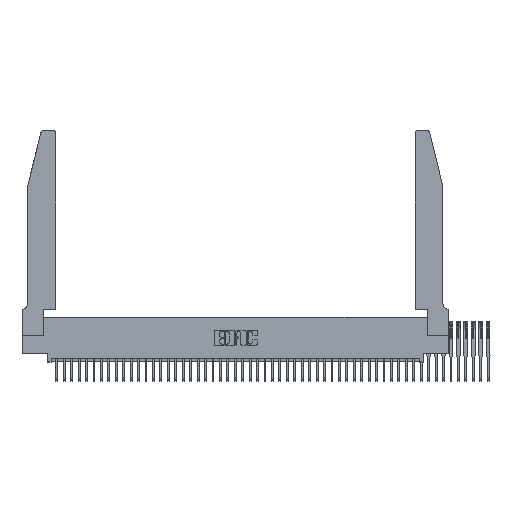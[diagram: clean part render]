
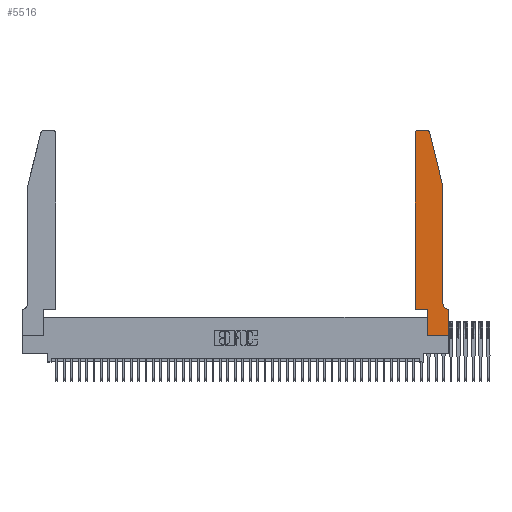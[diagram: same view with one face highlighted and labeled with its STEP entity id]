
A CAD part, top view. The second image highlights one B-rep face of the part: STEP entity #5516.
In plain terms, the highlighted face is planar.
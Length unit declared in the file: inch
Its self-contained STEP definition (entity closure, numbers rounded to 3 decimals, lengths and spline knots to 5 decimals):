
#220 = VERTEX_POINT ( 'NONE', #24858 ) ;
#544 = VERTEX_POINT ( 'NONE', #23576 ) ;
#2087 = EDGE_CURVE ( 'NONE', #5061, #9962, #10847, .T. ) ;
#2173 = DIRECTION ( 'NONE',  ( -1., 0., 0. ) ) ;
#2251 = CARTESIAN_POINT ( 'NONE',  ( 0.4505, 0.35, 0. ) ) ;
#2755 = VECTOR ( 'NONE', #5477, 39.37008 ) ;
#3337 = CARTESIAN_POINT ( 'NONE',  ( 0.2865, 0., 0. ) ) ;
#3999 = VERTEX_POINT ( 'NONE', #5056 ) ;
#4357 = ORIENTED_EDGE ( 'NONE', *, *, #26189, .F. ) ;
#4587 = LINE ( 'NONE', #8220, #20550 ) ;
#4733 = CARTESIAN_POINT ( 'NONE',  ( 0., 0., 0. ) ) ;
#4996 = CARTESIAN_POINT ( 'NONE',  ( 0.4205, 2.72, 0. ) ) ;
#5056 = CARTESIAN_POINT ( 'NONE',  ( 0.0755, 2., 0. ) ) ;
#5061 = VERTEX_POINT ( 'NONE', #17221 ) ;
#5477 = DIRECTION ( 'NONE',  ( 0., -1., 0. ) ) ;
#5516 = ADVANCED_FACE ( 'NONE', ( #7549 ), #6612, .F. ) ;
#6612 = PLANE ( 'NONE',  #25225 ) ;
#7189 = EDGE_LOOP ( 'NONE', ( #4357, #15729, #34381, #23136, #30529, #14920, #31548, #18931, #24250, #10706, #17897, #14163 ) ) ;
#7255 = EDGE_CURVE ( 'NONE', #27417, #16409, #16512, .T. ) ;
#7549 = FACE_OUTER_BOUND ( 'NONE', #7189, .T. ) ;
#7621 = CARTESIAN_POINT ( 'NONE',  ( 0.4205, 2.75, 0. ) ) ;
#8183 = DIRECTION ( 'NONE',  ( 1., 0., 0. ) ) ;
#8220 = CARTESIAN_POINT ( 'NONE',  ( 0.2865, 0.35, 0. ) ) ;
#9326 = VECTOR ( 'NONE', #34107, 39.37008 ) ;
#9565 = AXIS2_PLACEMENT_3D ( 'NONE', #28928, #9803, #32117 ) ;
#9674 = CIRCLE ( 'NONE', #20425, 0.03 ) ;
#9803 = DIRECTION ( 'NONE',  ( 0., 0., -1. ) ) ;
#9828 = VECTOR ( 'NONE', #23799, 39.37008 ) ;
#9962 = VERTEX_POINT ( 'NONE', #3337 ) ;
#10342 = LINE ( 'NONE', #18226, #9326 ) ;
#10705 = VERTEX_POINT ( 'NONE', #17101 ) ;
#10706 = ORIENTED_EDGE ( 'NONE', *, *, #17600, .F. ) ;
#10815 = CARTESIAN_POINT ( 'NONE',  ( 0.2605, 2.75, 0. ) ) ;
#10847 = LINE ( 'NONE', #4733, #9828 ) ;
#10950 = DIRECTION ( 'NONE',  ( -1., 0., 0. ) ) ;
#11025 = CIRCLE ( 'NONE', #15879, 0.03 ) ;
#11145 = EDGE_CURVE ( 'NONE', #220, #544, #27581, .T. ) ;
#12424 = DIRECTION ( 'NONE',  ( -0.239, -0.971, 0. ) ) ;
#14163 = ORIENTED_EDGE ( 'NONE', *, *, #37952, .F. ) ;
#14920 = ORIENTED_EDGE ( 'NONE', *, *, #36070, .F. ) ;
#15515 = VECTOR ( 'NONE', #2173, 39.37008 ) ;
#15729 = ORIENTED_EDGE ( 'NONE', *, *, #29593, .T. ) ;
#15879 = AXIS2_PLACEMENT_3D ( 'NONE', #4996, #27288, #8183 ) ;
#16221 = DIRECTION ( 'NONE',  ( 1., 0., 0. ) ) ;
#16409 = VERTEX_POINT ( 'NONE', #28227 ) ;
#16512 = LINE ( 'NONE', #10815, #31461 ) ;
#17101 = CARTESIAN_POINT ( 'NONE',  ( 0.25487, 2.72718, 0. ) ) ;
#17221 = CARTESIAN_POINT ( 'NONE',  ( 0., 0., 0. ) ) ;
#17463 = CARTESIAN_POINT ( 'NONE',  ( 0.2865, 0.35, 0. ) ) ;
#17544 = EDGE_CURVE ( 'NONE', #27417, #18672, #11025, .T. ) ;
#17600 = EDGE_CURVE ( 'NONE', #544, #26877, #40834, .T. ) ;
#17851 = DIRECTION ( 'NONE',  ( 1., 0., 0. ) ) ;
#17897 = ORIENTED_EDGE ( 'NONE', *, *, #11145, .F. ) ;
#18226 = CARTESIAN_POINT ( 'NONE',  ( 0.4505, 0.35, 0. ) ) ;
#18672 = VERTEX_POINT ( 'NONE', #20845 ) ;
#18931 = ORIENTED_EDGE ( 'NONE', *, *, #2087, .F. ) ;
#19003 = DIRECTION ( 'NONE',  ( 0., 0., -1. ) ) ;
#19398 = EDGE_CURVE ( 'NONE', #9962, #39148, #4587, .T. ) ;
#19434 = VECTOR ( 'NONE', #30331, 39.37008 ) ;
#19987 = VECTOR ( 'NONE', #12424, 39.37008 ) ;
#20425 = AXIS2_PLACEMENT_3D ( 'NONE', #38052, #19003, #41212 ) ;
#20550 = VECTOR ( 'NONE', #21074, 39.37008 ) ;
#20845 = CARTESIAN_POINT ( 'NONE',  ( 0.4505, 2.72, 0. ) ) ;
#21074 = DIRECTION ( 'NONE',  ( 0., 1., 0. ) ) ;
#21909 = EDGE_CURVE ( 'NONE', #34590, #18672, #10342, .T. ) ;
#23136 = ORIENTED_EDGE ( 'NONE', *, *, #17544, .T. ) ;
#23576 = CARTESIAN_POINT ( 'NONE',  ( 0.0055, 0.35, 0. ) ) ;
#23781 = CARTESIAN_POINT ( 'NONE',  ( 0., 0., 0. ) ) ;
#23799 = DIRECTION ( 'NONE',  ( 1., 0., 0. ) ) ;
#24250 = ORIENTED_EDGE ( 'NONE', *, *, #32529, .F. ) ;
#24858 = CARTESIAN_POINT ( 'NONE',  ( 0.0755, 0.42, 0. ) ) ;
#25225 = AXIS2_PLACEMENT_3D ( 'NONE', #32098, #35268, #16221 ) ;
#26131 = LINE ( 'NONE', #33729, #33562 ) ;
#26189 = EDGE_CURVE ( 'NONE', #10705, #3999, #28455, .T. ) ;
#26877 = VERTEX_POINT ( 'NONE', #39869 ) ;
#27288 = DIRECTION ( 'NONE',  ( 0., 0., -1. ) ) ;
#27417 = VERTEX_POINT ( 'NONE', #7621 ) ;
#27581 = CIRCLE ( 'NONE', #9565, 0.07 ) ;
#28227 = CARTESIAN_POINT ( 'NONE',  ( 0.284, 2.75, 0. ) ) ;
#28455 = LINE ( 'NONE', #34532, #19987 ) ;
#28928 = CARTESIAN_POINT ( 'NONE',  ( 0.0055, 0.42, 0. ) ) ;
#28932 = LINE ( 'NONE', #23781, #19434 ) ;
#29593 = EDGE_CURVE ( 'NONE', #10705, #16409, #9674, .T. ) ;
#30331 = DIRECTION ( 'NONE',  ( 0., -1., 0. ) ) ;
#30529 = ORIENTED_EDGE ( 'NONE', *, *, #21909, .F. ) ;
#31461 = VECTOR ( 'NONE', #10950, 39.37008 ) ;
#31548 = ORIENTED_EDGE ( 'NONE', *, *, #19398, .F. ) ;
#32098 = CARTESIAN_POINT ( 'NONE',  ( 0., 0.35, 0. ) ) ;
#32117 = DIRECTION ( 'NONE',  ( -1., 0., 0. ) ) ;
#32529 = EDGE_CURVE ( 'NONE', #26877, #5061, #28932, .T. ) ;
#33562 = VECTOR ( 'NONE', #17851, 39.37008 ) ;
#33729 = CARTESIAN_POINT ( 'NONE',  ( 0.4505, 0.35, 0. ) ) ;
#34107 = DIRECTION ( 'NONE',  ( 0., 1., 0. ) ) ;
#34381 = ORIENTED_EDGE ( 'NONE', *, *, #7255, .F. ) ;
#34532 = CARTESIAN_POINT ( 'NONE',  ( 0.0755, 2., 0. ) ) ;
#34590 = VERTEX_POINT ( 'NONE', #2251 ) ;
#35268 = DIRECTION ( 'NONE',  ( 0., 0., 1. ) ) ;
#35644 = LINE ( 'NONE', #40328, #2755 ) ;
#36070 = EDGE_CURVE ( 'NONE', #39148, #34590, #26131, .T. ) ;
#37952 = EDGE_CURVE ( 'NONE', #3999, #220, #35644, .T. ) ;
#38052 = CARTESIAN_POINT ( 'NONE',  ( 0.284, 2.72, 0. ) ) ;
#39148 = VERTEX_POINT ( 'NONE', #17463 ) ;
#39869 = CARTESIAN_POINT ( 'NONE',  ( 0., 0.35, 0. ) ) ;
#40267 = CARTESIAN_POINT ( 'NONE',  ( 0.0755, 0.35, 0. ) ) ;
#40328 = CARTESIAN_POINT ( 'NONE',  ( 0.0755, 2., 0. ) ) ;
#40834 = LINE ( 'NONE', #40267, #15515 ) ;
#41212 = DIRECTION ( 'NONE',  ( 1., 0., 0. ) ) ;
